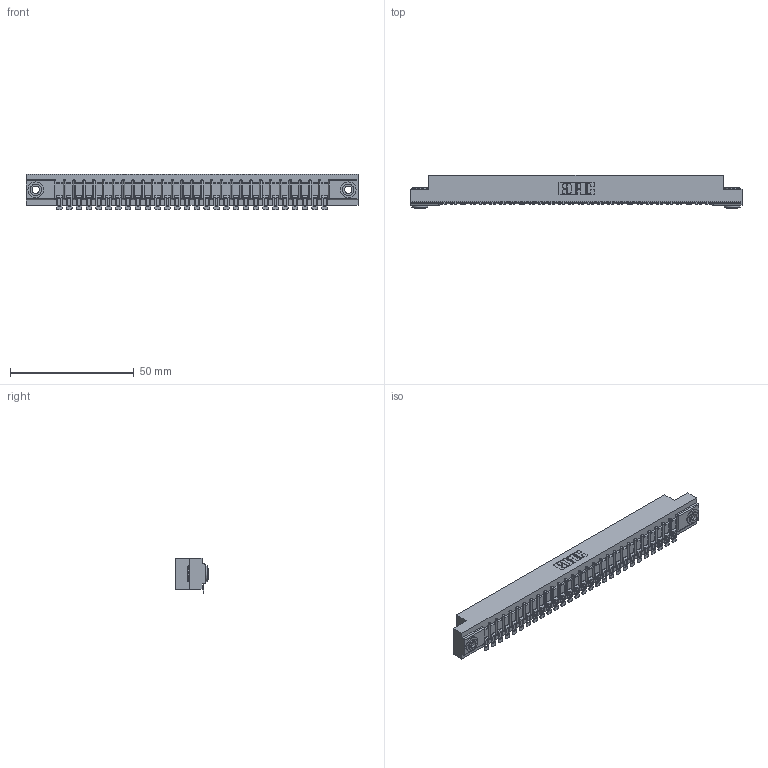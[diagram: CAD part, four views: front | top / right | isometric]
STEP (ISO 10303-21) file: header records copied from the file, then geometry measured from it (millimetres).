
FILE_DESCRIPTION (( 'STEP AP203' ), '1' );
FILE_NAME ('307-028-454-103.STEP', '2020-09-28T07:49:48', ( '' ), ( '' ), 'SwSTEP 2.0', 'SolidWorks 2020', '' );
FILE_SCHEMA (( 'CONFIG_CONTROL_DESIGN' ));
Length unit declared in the file: inch
Products named in the file (4): 307-028-454-103; 307-290-002_554; 345-250-002_345-250-002-102; 307 Part_.156 Dia Mounting Holes
Assembly tree (31 placements, depth 2):
  307-028-454-103
    307 Part_.156 Dia Mounting Holes
    307-290-002_554  x28
    345-250-002_345-250-002-102  x2
Bounding box: 133.96 x 13.36 x 14.52 mm (x, y, z)
Volume: 14242.4 mm3; surface area: 17958.4 mm2
Topology: 31 solids, 31 shells, 2467 faces, 7519 edges, 4930 vertices
Faces by surface type: plane 1382, cylinder 1019, sphere 58, cone 8
Entity records: 27760 total; most frequent: CARTESIAN_POINT 4659, ORIENTED_EDGE 4640, DIRECTION 4554, EDGE_CURVE 2320, VECTOR 1756, LINE 1756, VERTEX_POINT 1504, AXIS2_PLACEMENT_3D 1399
